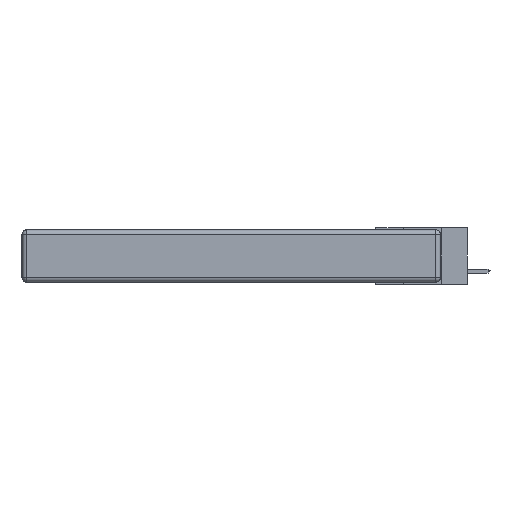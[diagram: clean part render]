
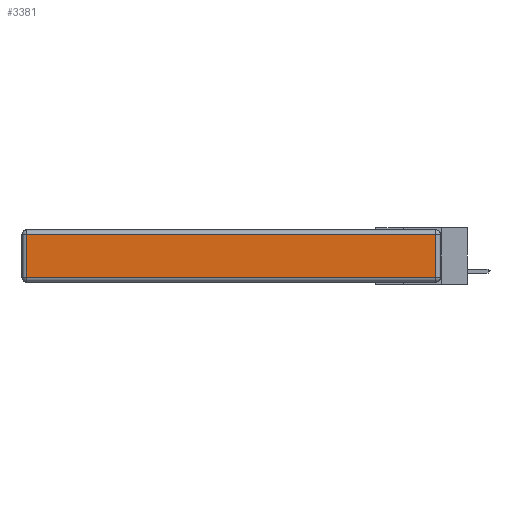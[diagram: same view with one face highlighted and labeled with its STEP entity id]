
A CAD part, left-side view. The second image highlights one B-rep face of the part: STEP entity #3381.
In plain terms, the highlighted planar face has unit normal (-1, 0, 0).
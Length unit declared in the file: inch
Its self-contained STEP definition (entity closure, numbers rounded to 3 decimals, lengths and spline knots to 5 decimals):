
#125 = VECTOR ( 'NONE', #30726, 39.37008 ) ;
#3381 = ADVANCED_FACE ( 'NONE', ( #23525 ), #4204, .T. ) ;
#4204 = PLANE ( 'NONE',  #21549 ) ;
#4925 = VECTOR ( 'NONE', #24369, 39.37008 ) ;
#5970 = EDGE_CURVE ( 'NONE', #6987, #29333, #15475, .T. ) ;
#6632 = CARTESIAN_POINT ( 'NONE',  ( 0., 0., -0.343 ) ) ;
#6987 = VERTEX_POINT ( 'NONE', #7198 ) ;
#7198 = CARTESIAN_POINT ( 'NONE',  ( 0., 0.03, -0.313 ) ) ;
#8366 = CARTESIAN_POINT ( 'NONE',  ( 0., 0.03, -0.03 ) ) ;
#9969 = CARTESIAN_POINT ( 'NONE',  ( 0., 0., -0.313 ) ) ;
#10748 = DIRECTION ( 'NONE',  ( 0., 1., 0. ) ) ;
#11522 = ORIENTED_EDGE ( 'NONE', *, *, #19001, .T. ) ;
#11787 = EDGE_LOOP ( 'NONE', ( #11799, #20946, #23452, #11522 ) ) ;
#11799 = ORIENTED_EDGE ( 'NONE', *, *, #27322, .T. ) ;
#14530 = LINE ( 'NONE', #18179, #125 ) ;
#15475 = LINE ( 'NONE', #29226, #4925 ) ;
#17353 = DIRECTION ( 'NONE',  ( 0., -1., 0. ) ) ;
#18179 = CARTESIAN_POINT ( 'NONE',  ( 0., 2.72, -0.343 ) ) ;
#18603 = LINE ( 'NONE', #9969, #24910 ) ;
#18911 = LINE ( 'NONE', #26325, #29419 ) ;
#19001 = EDGE_CURVE ( 'NONE', #29578, #26724, #14530, .T. ) ;
#19197 = CARTESIAN_POINT ( 'NONE',  ( 0., 2.72, -0.03 ) ) ;
#20946 = ORIENTED_EDGE ( 'NONE', *, *, #5970, .T. ) ;
#21450 = DIRECTION ( 'NONE',  ( 0., 0., 1. ) ) ;
#21549 = AXIS2_PLACEMENT_3D ( 'NONE', #6632, #31343, #21450 ) ;
#22238 = CARTESIAN_POINT ( 'NONE',  ( 0., 2.72, -0.313 ) ) ;
#23452 = ORIENTED_EDGE ( 'NONE', *, *, #28318, .T. ) ;
#23525 = FACE_OUTER_BOUND ( 'NONE', #11787, .T. ) ;
#24369 = DIRECTION ( 'NONE',  ( 0., 0., 1. ) ) ;
#24910 = VECTOR ( 'NONE', #17353, 39.37008 ) ;
#26325 = CARTESIAN_POINT ( 'NONE',  ( 0., 2.75, -0.03 ) ) ;
#26724 = VERTEX_POINT ( 'NONE', #22238 ) ;
#27322 = EDGE_CURVE ( 'NONE', #26724, #6987, #18603, .T. ) ;
#28318 = EDGE_CURVE ( 'NONE', #29333, #29578, #18911, .T. ) ;
#29226 = CARTESIAN_POINT ( 'NONE',  ( 0., 0.03, -0.343 ) ) ;
#29333 = VERTEX_POINT ( 'NONE', #8366 ) ;
#29419 = VECTOR ( 'NONE', #10748, 39.37008 ) ;
#29578 = VERTEX_POINT ( 'NONE', #19197 ) ;
#30726 = DIRECTION ( 'NONE',  ( 0., 0., -1. ) ) ;
#31343 = DIRECTION ( 'NONE',  ( -1., 0., 0. ) ) ;
